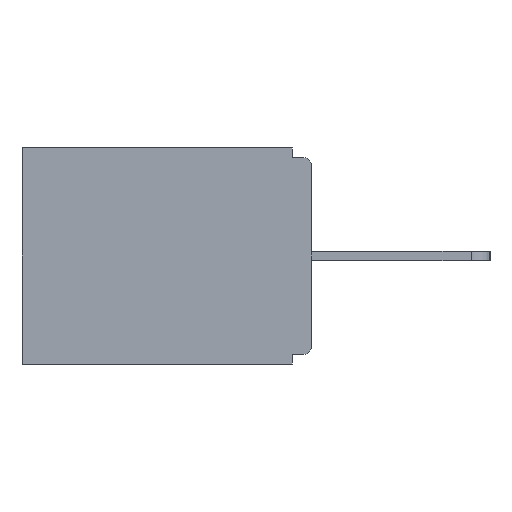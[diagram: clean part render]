
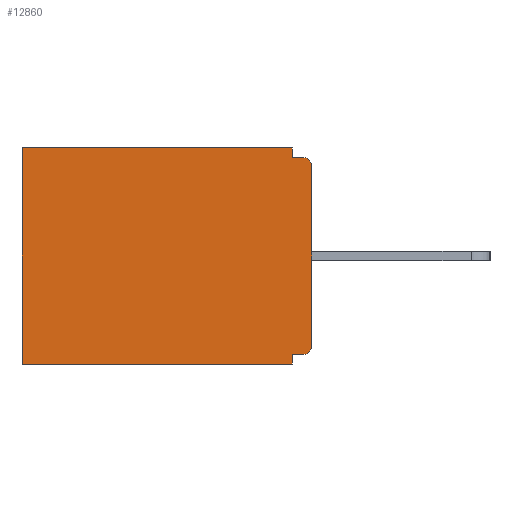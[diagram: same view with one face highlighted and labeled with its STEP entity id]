
A CAD part, left-side view. The second image highlights one B-rep face of the part: STEP entity #12860.
In plain terms, the highlighted planar face has unit normal (-1, 0, 0).
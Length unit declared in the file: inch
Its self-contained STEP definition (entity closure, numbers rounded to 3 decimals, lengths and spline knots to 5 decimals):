
#49 = VECTOR ( 'NONE', #18810, 39.37008 ) ;
#121 = VERTEX_POINT ( 'NONE', #9961 ) ;
#487 = DIRECTION ( 'NONE',  ( 0., 0., -1. ) ) ;
#733 = VERTEX_POINT ( 'NONE', #11429 ) ;
#894 = VERTEX_POINT ( 'NONE', #10138 ) ;
#1307 = CARTESIAN_POINT ( 'NONE',  ( 0.298, 0., 0. ) ) ;
#1726 = CIRCLE ( 'NONE', #9539, 0.015 ) ;
#1846 = CARTESIAN_POINT ( 'NONE',  ( 0.298, 0.031, -0.015 ) ) ;
#1939 = LINE ( 'NONE', #19009, #4762 ) ;
#2071 = VERTEX_POINT ( 'NONE', #2862 ) ;
#2453 = DIRECTION ( 'NONE',  ( 0., 1., 0. ) ) ;
#2500 = CARTESIAN_POINT ( 'NONE',  ( 0.298, 0.46, -0.343 ) ) ;
#2636 = EDGE_LOOP ( 'NONE', ( #7623, #6183, #9356, #3664, #20556, #17758, #13529, #17754, #20282, #14253 ) ) ;
#2803 = AXIS2_PLACEMENT_3D ( 'NONE', #8316, #19290, #9964 ) ;
#2829 = EDGE_CURVE ( 'NONE', #8049, #9076, #12568, .T. ) ;
#2846 = CIRCLE ( 'NONE', #2803, 0.015 ) ;
#2862 = CARTESIAN_POINT ( 'NONE',  ( 0.298, 0.031, -0.343 ) ) ;
#3664 = ORIENTED_EDGE ( 'NONE', *, *, #10250, .T. ) ;
#4060 = VERTEX_POINT ( 'NONE', #19176 ) ;
#4090 = CARTESIAN_POINT ( 'NONE',  ( 0.298, 0., 0. ) ) ;
#4477 = AXIS2_PLACEMENT_3D ( 'NONE', #18877, #9513, #20442 ) ;
#4762 = VECTOR ( 'NONE', #8027, 39.37008 ) ;
#5916 = DIRECTION ( 'NONE',  ( 0., 1., 0. ) ) ;
#5970 = EDGE_CURVE ( 'NONE', #8235, #894, #18818, .T. ) ;
#6114 = FACE_OUTER_BOUND ( 'NONE', #2636, .T. ) ;
#6131 = CARTESIAN_POINT ( 'NONE',  ( 0.298, 0.031, -0.343 ) ) ;
#6183 = ORIENTED_EDGE ( 'NONE', *, *, #14719, .F. ) ;
#6340 = EDGE_CURVE ( 'NONE', #2071, #8203, #20242, .T. ) ;
#6720 = VECTOR ( 'NONE', #5916, 39.37008 ) ;
#6880 = EDGE_CURVE ( 'NONE', #121, #733, #18289, .T. ) ;
#6947 = CARTESIAN_POINT ( 'NONE',  ( 0.298, 0.46, 0. ) ) ;
#7051 = LINE ( 'NONE', #4090, #15472 ) ;
#7623 = ORIENTED_EDGE ( 'NONE', *, *, #18817, .T. ) ;
#7813 = VECTOR ( 'NONE', #15823, 39.37008 ) ;
#8027 = DIRECTION ( 'NONE',  ( 0., -1., 0. ) ) ;
#8049 = VERTEX_POINT ( 'NONE', #12820 ) ;
#8086 = EDGE_CURVE ( 'NONE', #733, #2071, #16056, .T. ) ;
#8126 = DIRECTION ( 'NONE',  ( -1., 0., 0. ) ) ;
#8203 = VERTEX_POINT ( 'NONE', #2500 ) ;
#8235 = VERTEX_POINT ( 'NONE', #19440 ) ;
#8316 = CARTESIAN_POINT ( 'NONE',  ( 0.298, 0.015, -0.03 ) ) ;
#9076 = VERTEX_POINT ( 'NONE', #1846 ) ;
#9356 = ORIENTED_EDGE ( 'NONE', *, *, #2829, .F. ) ;
#9513 = DIRECTION ( 'NONE',  ( 1., 0., 0. ) ) ;
#9539 = AXIS2_PLACEMENT_3D ( 'NONE', #17559, #8126, #19103 ) ;
#9932 = EDGE_CURVE ( 'NONE', #121, #894, #1726, .T. ) ;
#9961 = CARTESIAN_POINT ( 'NONE',  ( 0.298, 0.015, -0.328 ) ) ;
#9964 = DIRECTION ( 'NONE',  ( 0., 0., -1. ) ) ;
#10138 = CARTESIAN_POINT ( 'NONE',  ( 0.298, 0., -0.313 ) ) ;
#10250 = EDGE_CURVE ( 'NONE', #8049, #4060, #7051, .T. ) ;
#10877 = CARTESIAN_POINT ( 'NONE',  ( 0.298, 0., -0.328 ) ) ;
#11429 = CARTESIAN_POINT ( 'NONE',  ( 0.298, 0.031, -0.328 ) ) ;
#12091 = VERTEX_POINT ( 'NONE', #18494 ) ;
#12568 = LINE ( 'NONE', #6131, #7813 ) ;
#12625 = DIRECTION ( 'NONE',  ( 0., 0., -1. ) ) ;
#12635 = PLANE ( 'NONE',  #4477 ) ;
#12820 = CARTESIAN_POINT ( 'NONE',  ( 0.298, 0.031, 0. ) ) ;
#12860 = ADVANCED_FACE ( 'NONE', ( #6114 ), #12635, .F. ) ;
#13529 = ORIENTED_EDGE ( 'NONE', *, *, #8086, .F. ) ;
#14253 = ORIENTED_EDGE ( 'NONE', *, *, #5970, .F. ) ;
#14719 = EDGE_CURVE ( 'NONE', #9076, #12091, #1939, .T. ) ;
#14723 = VECTOR ( 'NONE', #12625, 39.37008 ) ;
#15139 = VECTOR ( 'NONE', #487, 39.37008 ) ;
#15472 = VECTOR ( 'NONE', #2453, 39.37008 ) ;
#15823 = DIRECTION ( 'NONE',  ( 0., 0., -1. ) ) ;
#16056 = LINE ( 'NONE', #19480, #49 ) ;
#16133 = VECTOR ( 'NONE', #17515, 39.37008 ) ;
#17325 = EDGE_CURVE ( 'NONE', #4060, #8203, #19227, .T. ) ;
#17515 = DIRECTION ( 'NONE',  ( 0., 1., 0. ) ) ;
#17559 = CARTESIAN_POINT ( 'NONE',  ( 0.298, 0.015, -0.313 ) ) ;
#17754 = ORIENTED_EDGE ( 'NONE', *, *, #6880, .F. ) ;
#17758 = ORIENTED_EDGE ( 'NONE', *, *, #6340, .F. ) ;
#18289 = LINE ( 'NONE', #10877, #6720 ) ;
#18494 = CARTESIAN_POINT ( 'NONE',  ( 0.298, 0.015, -0.015 ) ) ;
#18810 = DIRECTION ( 'NONE',  ( 0., 0., -1. ) ) ;
#18817 = EDGE_CURVE ( 'NONE', #8235, #12091, #2846, .T. ) ;
#18818 = LINE ( 'NONE', #1307, #14723 ) ;
#18877 = CARTESIAN_POINT ( 'NONE',  ( 0.298, 0., 0. ) ) ;
#19009 = CARTESIAN_POINT ( 'NONE',  ( 0.298, 0., -0.015 ) ) ;
#19063 = CARTESIAN_POINT ( 'NONE',  ( 0.298, 0., -0.343 ) ) ;
#19103 = DIRECTION ( 'NONE',  ( 0., 0., -1. ) ) ;
#19176 = CARTESIAN_POINT ( 'NONE',  ( 0.298, 0.46, 0. ) ) ;
#19227 = LINE ( 'NONE', #6947, #15139 ) ;
#19290 = DIRECTION ( 'NONE',  ( -1., 0., 0. ) ) ;
#19440 = CARTESIAN_POINT ( 'NONE',  ( 0.298, 0., -0.03 ) ) ;
#19480 = CARTESIAN_POINT ( 'NONE',  ( 0.298, 0.031, -0.343 ) ) ;
#20242 = LINE ( 'NONE', #19063, #16133 ) ;
#20282 = ORIENTED_EDGE ( 'NONE', *, *, #9932, .T. ) ;
#20442 = DIRECTION ( 'NONE',  ( 0., 0., -1. ) ) ;
#20556 = ORIENTED_EDGE ( 'NONE', *, *, #17325, .T. ) ;
